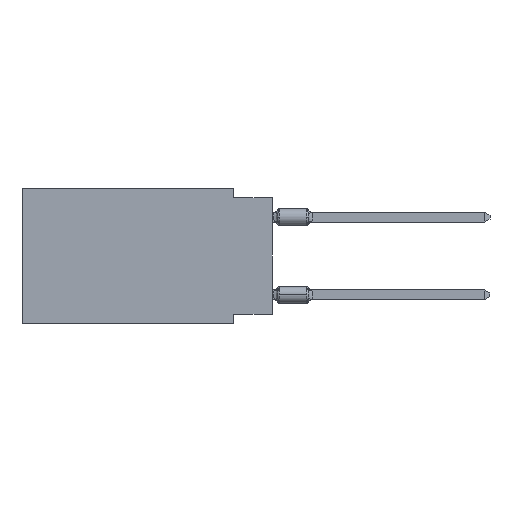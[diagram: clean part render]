
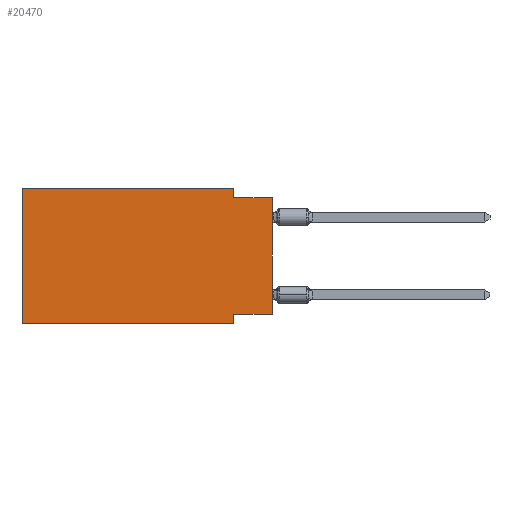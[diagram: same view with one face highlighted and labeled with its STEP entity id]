
A CAD part, left-side view. The second image highlights one B-rep face of the part: STEP entity #20470.
In plain terms, the highlighted planar face has unit normal (-1, 0, 0).
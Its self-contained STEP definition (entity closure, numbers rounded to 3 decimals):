
#105 = VECTOR ( 'NONE', #13920, 1000. ) ;
#131 = CARTESIAN_POINT ( 'NONE',  ( 0., 2.54, 0. ) ) ;
#194 = DIRECTION ( 'NONE',  ( 0., 0., 1. ) ) ;
#926 = CARTESIAN_POINT ( 'NONE',  ( 0., 0., -0.635 ) ) ;
#985 = CARTESIAN_POINT ( 'NONE',  ( 0., 2.54, -0.635 ) ) ;
#1203 = LINE ( 'NONE', #8582, #12500 ) ;
#1332 = VECTOR ( 'NONE', #194, 1000. ) ;
#1363 = CARTESIAN_POINT ( 'NONE',  ( 0., 16.383, 0. ) ) ;
#1452 = VERTEX_POINT ( 'NONE', #2358 ) ;
#1468 = VECTOR ( 'NONE', #20200, 1000. ) ;
#2358 = CARTESIAN_POINT ( 'NONE',  ( 0., 0., -8.255 ) ) ;
#3703 = VECTOR ( 'NONE', #18592, 1000. ) ;
#3860 = VECTOR ( 'NONE', #6325, 1000. ) ;
#4335 = LINE ( 'NONE', #11587, #3703 ) ;
#4502 = CARTESIAN_POINT ( 'NONE',  ( 0., 16.383, 0. ) ) ;
#4740 = DIRECTION ( 'NONE',  ( 1., 0., 0. ) ) ;
#5220 = VECTOR ( 'NONE', #20884, 1000. ) ;
#5846 = LINE ( 'NONE', #12966, #1468 ) ;
#5923 = EDGE_CURVE ( 'NONE', #10308, #22449, #21044, .T. ) ;
#6325 = DIRECTION ( 'NONE',  ( 0., 0., 1. ) ) ;
#6438 = CARTESIAN_POINT ( 'NONE',  ( 0., 16.383, -8.89 ) ) ;
#6663 = CARTESIAN_POINT ( 'NONE',  ( 0., 0., 0. ) ) ;
#7403 = EDGE_CURVE ( 'NONE', #16575, #10308, #23110, .T. ) ;
#7804 = CARTESIAN_POINT ( 'NONE',  ( 0., 2.54, 0. ) ) ;
#8582 = CARTESIAN_POINT ( 'NONE',  ( 0., 16.383, -8.89 ) ) ;
#9566 = EDGE_CURVE ( 'NONE', #19589, #10719, #1203, .T. ) ;
#9771 = DIRECTION ( 'NONE',  ( 0., 0., -1. ) ) ;
#10006 = FACE_OUTER_BOUND ( 'NONE', #13241, .T. ) ;
#10057 = CARTESIAN_POINT ( 'NONE',  ( 0., 2.54, -8.255 ) ) ;
#10308 = VERTEX_POINT ( 'NONE', #7804 ) ;
#10719 = VERTEX_POINT ( 'NONE', #16897 ) ;
#10809 = ORIENTED_EDGE ( 'NONE', *, *, #5923, .F. ) ;
#11054 = VECTOR ( 'NONE', #9771, 1000. ) ;
#11103 = ORIENTED_EDGE ( 'NONE', *, *, #13784, .F. ) ;
#11587 = CARTESIAN_POINT ( 'NONE',  ( 0., 0., -8.255 ) ) ;
#11752 = LINE ( 'NONE', #18758, #11054 ) ;
#12500 = VECTOR ( 'NONE', #15577, 1000. ) ;
#12966 = CARTESIAN_POINT ( 'NONE',  ( 0., 0., -0.635 ) ) ;
#13241 = EDGE_LOOP ( 'NONE', ( #15769, #20010, #10809, #19417, #16954, #13428, #18001, #11103 ) ) ;
#13263 = PLANE ( 'NONE',  #15186 ) ;
#13428 = ORIENTED_EDGE ( 'NONE', *, *, #9566, .T. ) ;
#13784 = EDGE_CURVE ( 'NONE', #1452, #19590, #4335, .T. ) ;
#13920 = DIRECTION ( 'NONE',  ( 0., 0., -1. ) ) ;
#15186 = AXIS2_PLACEMENT_3D ( 'NONE', #15248, #4740, #22381 ) ;
#15248 = CARTESIAN_POINT ( 'NONE',  ( 0., 16.383, 0. ) ) ;
#15577 = DIRECTION ( 'NONE',  ( 0., -1., 0. ) ) ;
#15769 = ORIENTED_EDGE ( 'NONE', *, *, #15829, .T. ) ;
#15829 = EDGE_CURVE ( 'NONE', #1452, #22074, #17292, .T. ) ;
#16575 = VERTEX_POINT ( 'NONE', #4502 ) ;
#16897 = CARTESIAN_POINT ( 'NONE',  ( 0., 2.54, -8.89 ) ) ;
#16954 = ORIENTED_EDGE ( 'NONE', *, *, #19056, .F. ) ;
#17292 = LINE ( 'NONE', #6663, #3860 ) ;
#18001 = ORIENTED_EDGE ( 'NONE', *, *, #19220, .F. ) ;
#18183 = LINE ( 'NONE', #21687, #1332 ) ;
#18592 = DIRECTION ( 'NONE',  ( 0., 1., 0. ) ) ;
#18758 = CARTESIAN_POINT ( 'NONE',  ( 0., 2.54, -8.89 ) ) ;
#19056 = EDGE_CURVE ( 'NONE', #19589, #16575, #18183, .T. ) ;
#19220 = EDGE_CURVE ( 'NONE', #19590, #10719, #11752, .T. ) ;
#19417 = ORIENTED_EDGE ( 'NONE', *, *, #7403, .F. ) ;
#19589 = VERTEX_POINT ( 'NONE', #6438 ) ;
#19590 = VERTEX_POINT ( 'NONE', #10057 ) ;
#20010 = ORIENTED_EDGE ( 'NONE', *, *, #21901, .F. ) ;
#20200 = DIRECTION ( 'NONE',  ( 0., -1., 0. ) ) ;
#20470 = ADVANCED_FACE ( 'NONE', ( #10006 ), #13263, .F. ) ;
#20884 = DIRECTION ( 'NONE',  ( 0., -1., 0. ) ) ;
#21044 = LINE ( 'NONE', #131, #105 ) ;
#21687 = CARTESIAN_POINT ( 'NONE',  ( 0., 16.383, 0. ) ) ;
#21901 = EDGE_CURVE ( 'NONE', #22449, #22074, #5846, .T. ) ;
#22074 = VERTEX_POINT ( 'NONE', #926 ) ;
#22381 = DIRECTION ( 'NONE',  ( 0., 0., -1. ) ) ;
#22449 = VERTEX_POINT ( 'NONE', #985 ) ;
#23110 = LINE ( 'NONE', #1363, #5220 ) ;
